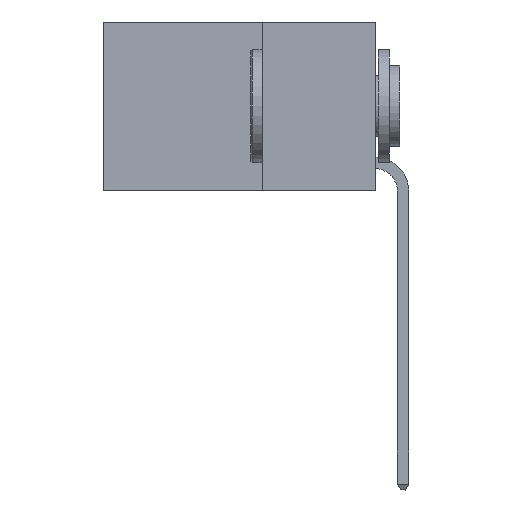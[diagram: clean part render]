
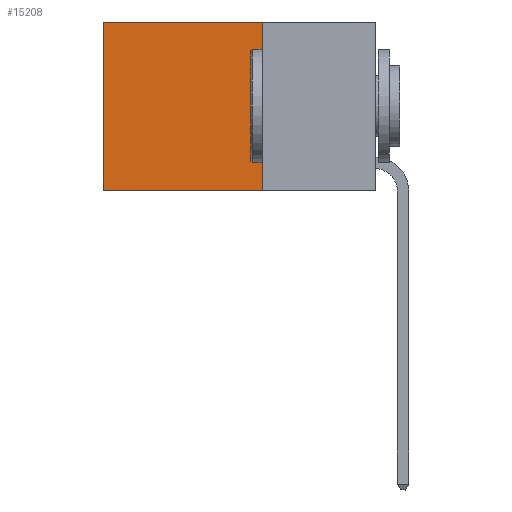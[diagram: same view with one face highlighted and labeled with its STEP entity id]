
A CAD part, left-side view. The second image highlights one B-rep face of the part: STEP entity #15208.
In plain terms, the highlighted planar face has unit normal (-1, 0, 0).
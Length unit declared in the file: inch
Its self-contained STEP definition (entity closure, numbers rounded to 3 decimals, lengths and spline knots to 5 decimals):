
#447 = ORIENTED_EDGE ( 'NONE', *, *, #19224, .T. ) ;
#848 = LINE ( 'NONE', #14374, #10491 ) ;
#1588 = DIRECTION ( 'NONE',  ( 0., 1., 0. ) ) ;
#1836 = VECTOR ( 'NONE', #12452, 39.37008 ) ;
#2601 = LINE ( 'NONE', #5954, #1836 ) ;
#2855 = CARTESIAN_POINT ( 'NONE',  ( 0.2625, 0.6, -0.37 ) ) ;
#4162 = DIRECTION ( 'NONE',  ( 0., 0., -1. ) ) ;
#4875 = EDGE_LOOP ( 'NONE', ( #447, #14954, #16591, #6846 ) ) ;
#5237 = DIRECTION ( 'NONE',  ( 0., 0., -1. ) ) ;
#5466 = PLANE ( 'NONE',  #16985 ) ;
#5710 = VERTEX_POINT ( 'NONE', #17067 ) ;
#5954 = CARTESIAN_POINT ( 'NONE',  ( 0.2625, 0.25, -0.37 ) ) ;
#6292 = VERTEX_POINT ( 'NONE', #18408 ) ;
#6846 = ORIENTED_EDGE ( 'NONE', *, *, #16382, .T. ) ;
#7428 = FACE_OUTER_BOUND ( 'NONE', #4875, .T. ) ;
#8646 = VECTOR ( 'NONE', #1588, 39.37008 ) ;
#9203 = VERTEX_POINT ( 'NONE', #2855 ) ;
#9599 = VERTEX_POINT ( 'NONE', #11150 ) ;
#10370 = DIRECTION ( 'NONE',  ( 1., 0., 0. ) ) ;
#10491 = VECTOR ( 'NONE', #4162, 39.37008 ) ;
#11150 = CARTESIAN_POINT ( 'NONE',  ( 0.2625, 0.6, 0. ) ) ;
#11433 = CARTESIAN_POINT ( 'NONE',  ( 0.2625, 0.25, 0. ) ) ;
#12452 = DIRECTION ( 'NONE',  ( 0., 1., 0. ) ) ;
#13266 = LINE ( 'NONE', #21372, #17689 ) ;
#14374 = CARTESIAN_POINT ( 'NONE',  ( 0.2625, 0.6, 0. ) ) ;
#14792 = LINE ( 'NONE', #11433, #8646 ) ;
#14954 = ORIENTED_EDGE ( 'NONE', *, *, #15840, .F. ) ;
#15208 = ADVANCED_FACE ( 'NONE', ( #7428 ), #5466, .F. ) ;
#15463 = EDGE_CURVE ( 'NONE', #5710, #6292, #13266, .T. ) ;
#15840 = EDGE_CURVE ( 'NONE', #6292, #9203, #2601, .T. ) ;
#16382 = EDGE_CURVE ( 'NONE', #5710, #9599, #14792, .T. ) ;
#16591 = ORIENTED_EDGE ( 'NONE', *, *, #15463, .F. ) ;
#16924 = DIRECTION ( 'NONE',  ( 0., 0., -1. ) ) ;
#16985 = AXIS2_PLACEMENT_3D ( 'NONE', #17354, #10370, #16924 ) ;
#17067 = CARTESIAN_POINT ( 'NONE',  ( 0.2625, 0.25, 0. ) ) ;
#17354 = CARTESIAN_POINT ( 'NONE',  ( 0.2625, 0.25, 0. ) ) ;
#17689 = VECTOR ( 'NONE', #5237, 39.37008 ) ;
#18408 = CARTESIAN_POINT ( 'NONE',  ( 0.2625, 0.25, -0.37 ) ) ;
#19224 = EDGE_CURVE ( 'NONE', #9599, #9203, #848, .T. ) ;
#21372 = CARTESIAN_POINT ( 'NONE',  ( 0.2625, 0.25, 0. ) ) ;
